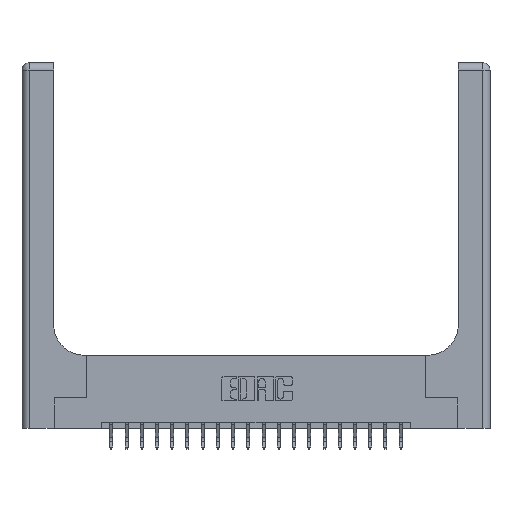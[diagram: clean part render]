
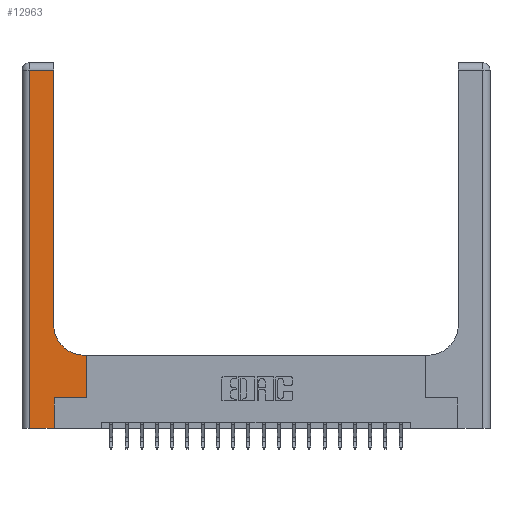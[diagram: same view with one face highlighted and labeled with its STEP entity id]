
A CAD part, top view. The second image highlights one B-rep face of the part: STEP entity #12963.
In plain terms, the highlighted planar face has unit normal (0, 0, 1).
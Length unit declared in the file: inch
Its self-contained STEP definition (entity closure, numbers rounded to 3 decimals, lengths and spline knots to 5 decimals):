
#173 = VERTEX_POINT ( 'NONE', #17307 ) ;
#450 = VECTOR ( 'NONE', #1511, 39.37008 ) ;
#953 = VERTEX_POINT ( 'NONE', #17229 ) ;
#1131 = CARTESIAN_POINT ( 'NONE',  ( 0.26, 0.6, 0.37 ) ) ;
#1163 = DIRECTION ( 'NONE',  ( -1., 0., 0. ) ) ;
#1360 = EDGE_CURVE ( 'NONE', #173, #21058, #8444, .T. ) ;
#1511 = DIRECTION ( 'NONE',  ( 0., -1., 0. ) ) ;
#2462 = ORIENTED_EDGE ( 'NONE', *, *, #6760, .T. ) ;
#3395 = CARTESIAN_POINT ( 'NONE',  ( 0., 3., 0.37 ) ) ;
#3399 = DIRECTION ( 'NONE',  ( 0., 1., 0. ) ) ;
#5035 = DIRECTION ( 'NONE',  ( 1., 0., 0. ) ) ;
#5142 = VERTEX_POINT ( 'NONE', #17010 ) ;
#5177 = PLANE ( 'NONE',  #6732 ) ;
#5750 = ORIENTED_EDGE ( 'NONE', *, *, #17209, .T. ) ;
#5919 = EDGE_CURVE ( 'NONE', #10064, #5142, #7030, .T. ) ;
#6087 = VERTEX_POINT ( 'NONE', #21821 ) ;
#6335 = LINE ( 'NONE', #1131, #14168 ) ;
#6555 = DIRECTION ( 'NONE',  ( 0., 0., -1. ) ) ;
#6732 = AXIS2_PLACEMENT_3D ( 'NONE', #3395, #16900, #17240 ) ;
#6760 = EDGE_CURVE ( 'NONE', #6087, #953, #16768, .T. ) ;
#6942 = FACE_OUTER_BOUND ( 'NONE', #10565, .T. ) ;
#7030 = CIRCLE ( 'NONE', #8813, 0.25 ) ;
#7051 = EDGE_CURVE ( 'NONE', #20778, #14652, #19298, .T. ) ;
#7127 = DIRECTION ( 'NONE',  ( 0., 1., 0. ) ) ;
#7680 = VECTOR ( 'NONE', #7685, 39.37008 ) ;
#7685 = DIRECTION ( 'NONE',  ( 0., 1., 0. ) ) ;
#7698 = VERTEX_POINT ( 'NONE', #21458 ) ;
#7870 = CARTESIAN_POINT ( 'NONE',  ( 0.51, 0.6, 0.37 ) ) ;
#7895 = DIRECTION ( 'NONE',  ( -1., 0., 0. ) ) ;
#8156 = CARTESIAN_POINT ( 'NONE',  ( 0.26, 3., 0.37 ) ) ;
#8232 = EDGE_CURVE ( 'NONE', #21058, #20778, #10003, .T. ) ;
#8444 = LINE ( 'NONE', #17310, #19151 ) ;
#8813 = AXIS2_PLACEMENT_3D ( 'NONE', #11296, #6555, #16625 ) ;
#9004 = ORIENTED_EDGE ( 'NONE', *, *, #14884, .T. ) ;
#9091 = VECTOR ( 'NONE', #1163, 39.37008 ) ;
#9668 = CARTESIAN_POINT ( 'NONE',  ( 0.528, 0.25, 0.37 ) ) ;
#9895 = CARTESIAN_POINT ( 'NONE',  ( 0.06, 3., 0.37 ) ) ;
#10003 = LINE ( 'NONE', #13410, #12634 ) ;
#10064 = VERTEX_POINT ( 'NONE', #7870 ) ;
#10565 = EDGE_LOOP ( 'NONE', ( #17572, #2462, #5750, #9004, #12547, #18177, #14691, #18521, #21471 ) ) ;
#10887 = CARTESIAN_POINT ( 'NONE',  ( 0., 0., 0.37 ) ) ;
#11269 = CARTESIAN_POINT ( 'NONE',  ( 0.265, 0.25, 0.37 ) ) ;
#11296 = CARTESIAN_POINT ( 'NONE',  ( 0.51, 0.85, 0.37 ) ) ;
#12547 = ORIENTED_EDGE ( 'NONE', *, *, #1360, .T. ) ;
#12634 = VECTOR ( 'NONE', #5035, 39.37008 ) ;
#12963 = ADVANCED_FACE ( 'NONE', ( #6942 ), #5177, .F. ) ;
#13410 = CARTESIAN_POINT ( 'NONE',  ( 0.265, 0.25, 0.37 ) ) ;
#13680 = DIRECTION ( 'NONE',  ( 1., 0., 0. ) ) ;
#13736 = EDGE_CURVE ( 'NONE', #14652, #10064, #6335, .T. ) ;
#14168 = VECTOR ( 'NONE', #7895, 39.37008 ) ;
#14204 = CARTESIAN_POINT ( 'NONE',  ( 0.528, 0.25, 0.37 ) ) ;
#14652 = VERTEX_POINT ( 'NONE', #15929 ) ;
#14691 = ORIENTED_EDGE ( 'NONE', *, *, #7051, .T. ) ;
#14786 = EDGE_CURVE ( 'NONE', #5142, #6087, #18566, .T. ) ;
#14884 = EDGE_CURVE ( 'NONE', #7698, #173, #17018, .T. ) ;
#14988 = CARTESIAN_POINT ( 'NONE',  ( 0., 2.94, 0.37 ) ) ;
#15929 = CARTESIAN_POINT ( 'NONE',  ( 0.528, 0.6, 0.37 ) ) ;
#16625 = DIRECTION ( 'NONE',  ( 1., 0., 0. ) ) ;
#16704 = VECTOR ( 'NONE', #3399, 39.37008 ) ;
#16768 = LINE ( 'NONE', #14988, #9091 ) ;
#16900 = DIRECTION ( 'NONE',  ( 0., 0., -1. ) ) ;
#17010 = CARTESIAN_POINT ( 'NONE',  ( 0.26, 0.85, 0.37 ) ) ;
#17018 = LINE ( 'NONE', #10887, #21643 ) ;
#17209 = EDGE_CURVE ( 'NONE', #953, #7698, #20533, .T. ) ;
#17229 = CARTESIAN_POINT ( 'NONE',  ( 0.06, 2.94, 0.37 ) ) ;
#17240 = DIRECTION ( 'NONE',  ( -1., 0., 0. ) ) ;
#17307 = CARTESIAN_POINT ( 'NONE',  ( 0.265, 0., 0.37 ) ) ;
#17310 = CARTESIAN_POINT ( 'NONE',  ( 0.265, 0., 0.37 ) ) ;
#17572 = ORIENTED_EDGE ( 'NONE', *, *, #14786, .T. ) ;
#18177 = ORIENTED_EDGE ( 'NONE', *, *, #8232, .T. ) ;
#18521 = ORIENTED_EDGE ( 'NONE', *, *, #13736, .T. ) ;
#18566 = LINE ( 'NONE', #8156, #16704 ) ;
#19151 = VECTOR ( 'NONE', #7127, 39.37008 ) ;
#19298 = LINE ( 'NONE', #14204, #7680 ) ;
#20533 = LINE ( 'NONE', #9895, #450 ) ;
#20778 = VERTEX_POINT ( 'NONE', #9668 ) ;
#21058 = VERTEX_POINT ( 'NONE', #11269 ) ;
#21458 = CARTESIAN_POINT ( 'NONE',  ( 0.06, 0., 0.37 ) ) ;
#21471 = ORIENTED_EDGE ( 'NONE', *, *, #5919, .T. ) ;
#21643 = VECTOR ( 'NONE', #13680, 39.37008 ) ;
#21821 = CARTESIAN_POINT ( 'NONE',  ( 0.26, 2.94, 0.37 ) ) ;
